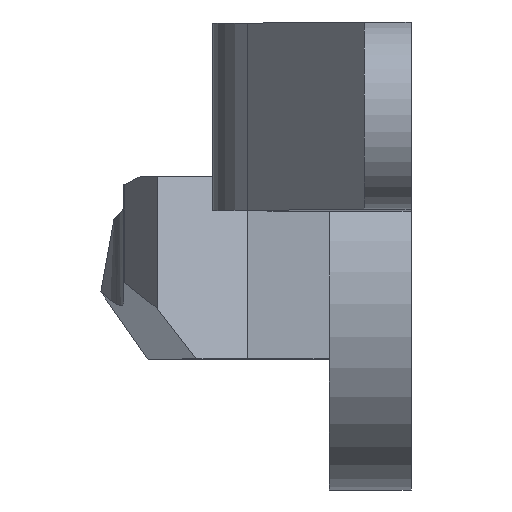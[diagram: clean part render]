
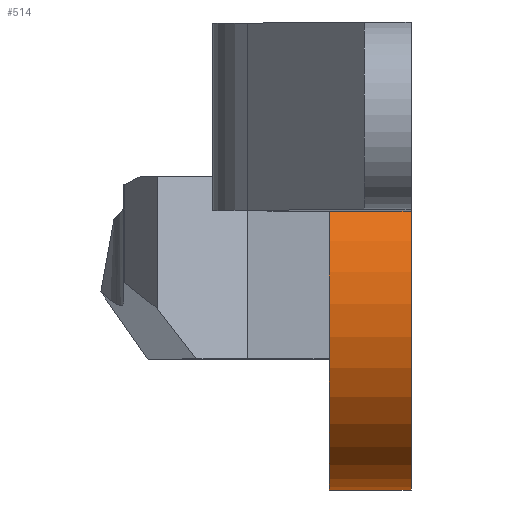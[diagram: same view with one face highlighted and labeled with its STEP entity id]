
A CAD part, top view. The second image highlights one B-rep face of the part: STEP entity #514.
In plain terms, the highlighted cylindrical face has radius 8 mm (diameter 16 mm), a partial arc.
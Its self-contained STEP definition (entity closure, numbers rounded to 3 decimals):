
#48 = CARTESIAN_POINT ( 'NONE',  ( 7., -5.759, -58.077 ) ) ;
#54 = VERTEX_POINT ( 'NONE', #65 ) ;
#55 = DIRECTION ( 'NONE',  ( 1., 0., 0. ) ) ;
#65 = CARTESIAN_POINT ( 'NONE',  ( 3.5, -1.852, -65.058 ) ) ;
#82 = ORIENTED_EDGE ( 'NONE', *, *, #475, .F. ) ;
#92 = AXIS2_PLACEMENT_3D ( 'NONE', #663, #660, #670 ) ;
#148 = CARTESIAN_POINT ( 'NONE',  ( 7., -1.852, -51.096 ) ) ;
#187 = EDGE_LOOP ( 'NONE', ( #82, #800, #898, #915 ) ) ;
#211 = VERTEX_POINT ( 'NONE', #637 ) ;
#234 = AXIS2_PLACEMENT_3D ( 'NONE', #48, #55, #367 ) ;
#269 = AXIS2_PLACEMENT_3D ( 'NONE', #820, #930, #485 ) ;
#367 = DIRECTION ( 'NONE',  ( 0., 0., -1. ) ) ;
#368 = LINE ( 'NONE', #888, #410 ) ;
#374 = VERTEX_POINT ( 'NONE', #148 ) ;
#404 = VECTOR ( 'NONE', #488, 1000. ) ;
#410 = VECTOR ( 'NONE', #825, 1000. ) ;
#420 = LINE ( 'NONE', #885, #404 ) ;
#475 = EDGE_CURVE ( 'NONE', #374, #211, #765, .T. ) ;
#485 = DIRECTION ( 'NONE',  ( 0., 0., -1. ) ) ;
#488 = DIRECTION ( 'NONE',  ( 1., 0., 0. ) ) ;
#514 = ADVANCED_FACE ( 'NONE', ( #785 ), #849, .T. ) ;
#588 = EDGE_CURVE ( 'NONE', #803, #54, #913, .T. ) ;
#637 = CARTESIAN_POINT ( 'NONE',  ( 7., -1.852, -65.058 ) ) ;
#660 = DIRECTION ( 'NONE',  ( 1., 0., 0. ) ) ;
#663 = CARTESIAN_POINT ( 'NONE',  ( 3.5, -5.759, -58.077 ) ) ;
#670 = DIRECTION ( 'NONE',  ( 0., 0., -1. ) ) ;
#765 = CIRCLE ( 'NONE', #234, 8. ) ;
#785 = FACE_OUTER_BOUND ( 'NONE', #187, .T. ) ;
#800 = ORIENTED_EDGE ( 'NONE', *, *, #886, .F. ) ;
#803 = VERTEX_POINT ( 'NONE', #858 ) ;
#820 = CARTESIAN_POINT ( 'NONE',  ( 3.5, -5.759, -58.077 ) ) ;
#825 = DIRECTION ( 'NONE',  ( 1., 0., 0. ) ) ;
#849 = CYLINDRICAL_SURFACE ( 'NONE', #92, 8. ) ;
#858 = CARTESIAN_POINT ( 'NONE',  ( 3.5, -1.852, -51.096 ) ) ;
#885 = CARTESIAN_POINT ( 'NONE',  ( 3.5, -1.852, -51.096 ) ) ;
#886 = EDGE_CURVE ( 'NONE', #803, #374, #420, .T. ) ;
#888 = CARTESIAN_POINT ( 'NONE',  ( 3.5, -1.852, -65.058 ) ) ;
#890 = EDGE_CURVE ( 'NONE', #54, #211, #368, .T. ) ;
#898 = ORIENTED_EDGE ( 'NONE', *, *, #588, .T. ) ;
#913 = CIRCLE ( 'NONE', #269, 8. ) ;
#915 = ORIENTED_EDGE ( 'NONE', *, *, #890, .T. ) ;
#930 = DIRECTION ( 'NONE',  ( 1., 0., 0. ) ) ;
